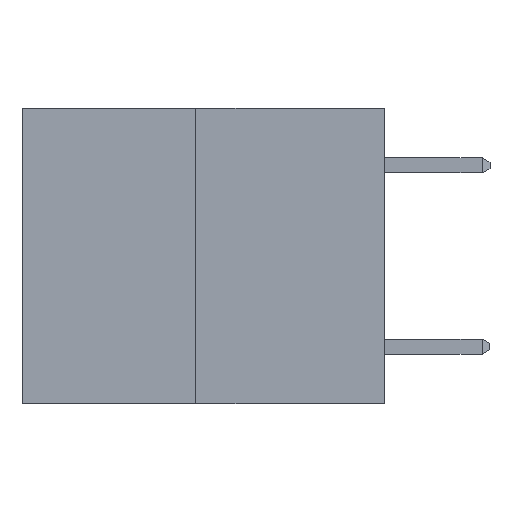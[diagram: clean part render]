
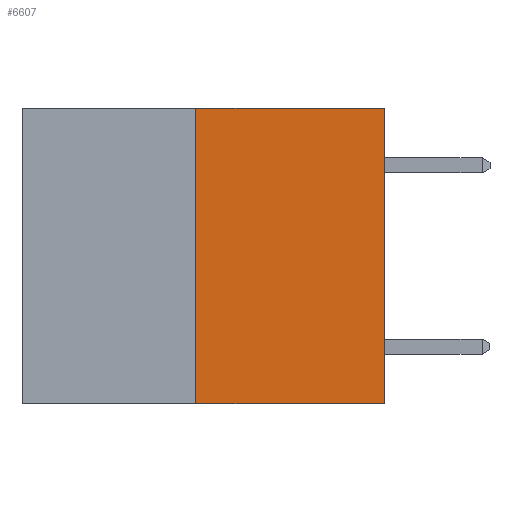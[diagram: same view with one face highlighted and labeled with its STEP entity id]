
A CAD part, left-side view. The second image highlights one B-rep face of the part: STEP entity #6607.
In plain terms, the highlighted planar face has unit normal (-1, 0, 0).
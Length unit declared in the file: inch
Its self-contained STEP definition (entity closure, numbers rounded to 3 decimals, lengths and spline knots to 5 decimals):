
#1216 = VECTOR ( 'NONE', #7564, 39.37008 ) ;
#1593 = EDGE_CURVE ( 'NONE', #3512, #16182, #15140, .T. ) ;
#2274 = CARTESIAN_POINT ( 'NONE',  ( 0., 0.6, 0. ) ) ;
#2853 = LINE ( 'NONE', #2274, #6338 ) ;
#3231 = LINE ( 'NONE', #15983, #12250 ) ;
#3321 = FACE_OUTER_BOUND ( 'NONE', #12278, .T. ) ;
#3414 = DIRECTION ( 'NONE',  ( 0., 0., 1. ) ) ;
#3512 = VERTEX_POINT ( 'NONE', #12010 ) ;
#3938 = CARTESIAN_POINT ( 'NONE',  ( 0., 0., -0.49 ) ) ;
#4003 = ORIENTED_EDGE ( 'NONE', *, *, #1593, .T. ) ;
#4320 = PLANE ( 'NONE',  #9989 ) ;
#6338 = VECTOR ( 'NONE', #7485, 39.37008 ) ;
#6607 = ADVANCED_FACE ( 'NONE', ( #3321 ), #4320, .F. ) ;
#7485 = DIRECTION ( 'NONE',  ( 0., -1., 0. ) ) ;
#7564 = DIRECTION ( 'NONE',  ( 0., -1., 0. ) ) ;
#7659 = CARTESIAN_POINT ( 'NONE',  ( 0., 0.312, 0. ) ) ;
#8293 = VECTOR ( 'NONE', #3414, 39.37008 ) ;
#8460 = DIRECTION ( 'NONE',  ( 0., 0., 1. ) ) ;
#9989 = AXIS2_PLACEMENT_3D ( 'NONE', #16115, #12333, #13580 ) ;
#10231 = EDGE_CURVE ( 'NONE', #16182, #13981, #3231, .T. ) ;
#10869 = CARTESIAN_POINT ( 'NONE',  ( 0., 0., 0. ) ) ;
#12010 = CARTESIAN_POINT ( 'NONE',  ( 0., 0.312, -0.49 ) ) ;
#12250 = VECTOR ( 'NONE', #8460, 39.37008 ) ;
#12278 = EDGE_LOOP ( 'NONE', ( #16805, #4003, #12743, #16786 ) ) ;
#12333 = DIRECTION ( 'NONE',  ( 1., 0., 0. ) ) ;
#12663 = EDGE_CURVE ( 'NONE', #3512, #16447, #12780, .T. ) ;
#12743 = ORIENTED_EDGE ( 'NONE', *, *, #10231, .T. ) ;
#12780 = LINE ( 'NONE', #15211, #8293 ) ;
#13580 = DIRECTION ( 'NONE',  ( 0., 0., -1. ) ) ;
#13981 = VERTEX_POINT ( 'NONE', #10869 ) ;
#14991 = EDGE_CURVE ( 'NONE', #16447, #13981, #2853, .T. ) ;
#15140 = LINE ( 'NONE', #15389, #1216 ) ;
#15211 = CARTESIAN_POINT ( 'NONE',  ( 0., 0.312, -0.49 ) ) ;
#15389 = CARTESIAN_POINT ( 'NONE',  ( 0., 0.6, -0.49 ) ) ;
#15983 = CARTESIAN_POINT ( 'NONE',  ( 0., 0., 0. ) ) ;
#16115 = CARTESIAN_POINT ( 'NONE',  ( 0., 0.6, 0. ) ) ;
#16182 = VERTEX_POINT ( 'NONE', #3938 ) ;
#16447 = VERTEX_POINT ( 'NONE', #7659 ) ;
#16786 = ORIENTED_EDGE ( 'NONE', *, *, #14991, .F. ) ;
#16805 = ORIENTED_EDGE ( 'NONE', *, *, #12663, .F. ) ;
